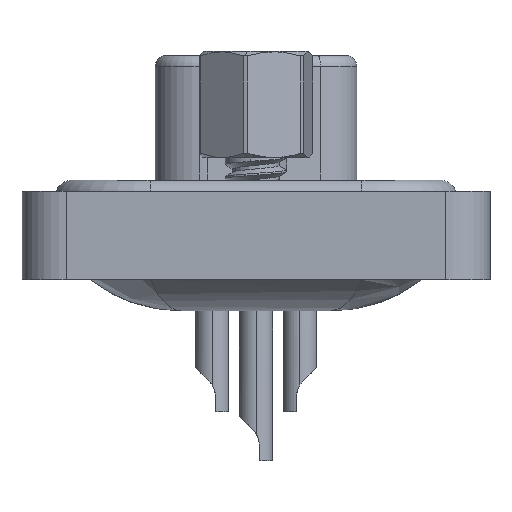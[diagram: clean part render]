
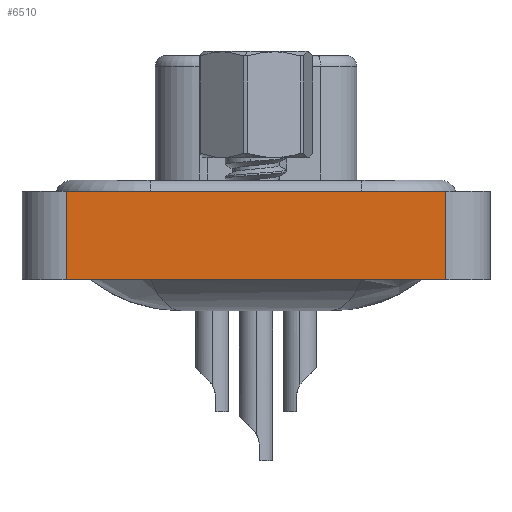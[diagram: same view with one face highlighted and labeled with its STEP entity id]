
A CAD part, left-side view. The second image highlights one B-rep face of the part: STEP entity #6510.
In plain terms, the highlighted planar face has unit normal (-1, 0, 0).
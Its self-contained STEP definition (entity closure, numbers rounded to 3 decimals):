
#549 = LINE ( 'NONE', #26720, #15794 ) ;
#555 = VECTOR ( 'NONE', #3414, 1000. ) ;
#1679 = CARTESIAN_POINT ( 'NONE',  ( -7.285, 8.55, -3.6 ) ) ;
#2018 = VERTEX_POINT ( 'NONE', #2781 ) ;
#2781 = CARTESIAN_POINT ( 'NONE',  ( -7.285, 8.55, 0.4 ) ) ;
#3024 = VERTEX_POINT ( 'NONE', #19843 ) ;
#3414 = DIRECTION ( 'NONE',  ( 0., -1., 0. ) ) ;
#4216 = LINE ( 'NONE', #1679, #5461 ) ;
#4223 = VERTEX_POINT ( 'NONE', #12142 ) ;
#4942 = CARTESIAN_POINT ( 'NONE',  ( -7.285, -8.55, -3.6 ) ) ;
#5461 = VECTOR ( 'NONE', #6195, 1000. ) ;
#6069 = EDGE_CURVE ( 'NONE', #2018, #4223, #549, .T. ) ;
#6195 = DIRECTION ( 'NONE',  ( 0., 0., 1. ) ) ;
#6510 = ADVANCED_FACE ( 'NONE', ( #24420 ), #11679, .T. ) ;
#7924 = EDGE_CURVE ( 'NONE', #23546, #2018, #4216, .T. ) ;
#8239 = CARTESIAN_POINT ( 'NONE',  ( -7.285, -8.55, -3.6 ) ) ;
#8291 = ORIENTED_EDGE ( 'NONE', *, *, #7924, .F. ) ;
#10824 = EDGE_CURVE ( 'NONE', #3024, #4223, #24350, .T. ) ;
#11205 = ORIENTED_EDGE ( 'NONE', *, *, #6069, .F. ) ;
#11679 = PLANE ( 'NONE',  #25755 ) ;
#11818 = DIRECTION ( 'NONE',  ( -1., 0., 0. ) ) ;
#12142 = CARTESIAN_POINT ( 'NONE',  ( -7.285, -8.55, 0.4 ) ) ;
#13607 = DIRECTION ( 'NONE',  ( 0., 0., 1. ) ) ;
#13673 = DIRECTION ( 'NONE',  ( 0., 0., 1. ) ) ;
#15794 = VECTOR ( 'NONE', #20347, 1000. ) ;
#16746 = LINE ( 'NONE', #8239, #555 ) ;
#17331 = EDGE_CURVE ( 'NONE', #23546, #3024, #16746, .T. ) ;
#18224 = EDGE_LOOP ( 'NONE', ( #18824, #11205, #8291, #25261 ) ) ;
#18824 = ORIENTED_EDGE ( 'NONE', *, *, #10824, .T. ) ;
#19843 = CARTESIAN_POINT ( 'NONE',  ( -7.285, -8.55, -3.6 ) ) ;
#20347 = DIRECTION ( 'NONE',  ( 0., -1., 0. ) ) ;
#20452 = CARTESIAN_POINT ( 'NONE',  ( -7.285, -8.55, -3.6 ) ) ;
#21997 = CARTESIAN_POINT ( 'NONE',  ( -7.285, 8.55, -3.6 ) ) ;
#23546 = VERTEX_POINT ( 'NONE', #21997 ) ;
#24350 = LINE ( 'NONE', #4942, #25277 ) ;
#24420 = FACE_OUTER_BOUND ( 'NONE', #18224, .T. ) ;
#25261 = ORIENTED_EDGE ( 'NONE', *, *, #17331, .T. ) ;
#25277 = VECTOR ( 'NONE', #13607, 1000. ) ;
#25755 = AXIS2_PLACEMENT_3D ( 'NONE', #20452, #11818, #13673 ) ;
#26720 = CARTESIAN_POINT ( 'NONE',  ( -7.285, -8.55, 0.4 ) ) ;
